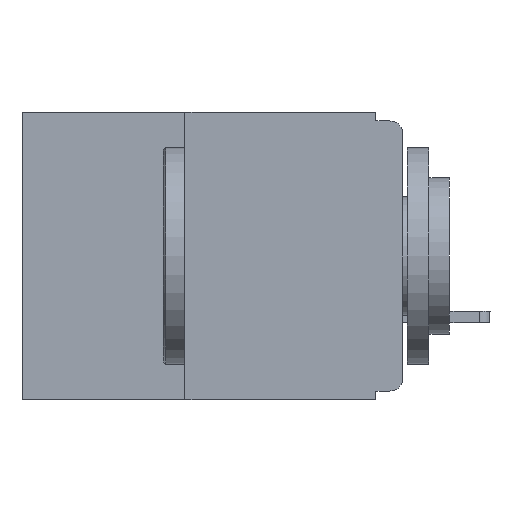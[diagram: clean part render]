
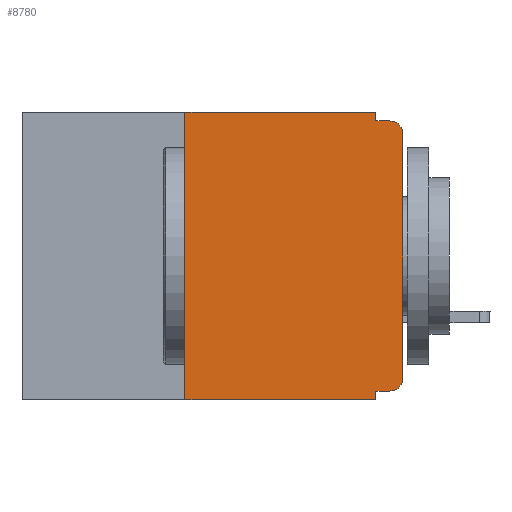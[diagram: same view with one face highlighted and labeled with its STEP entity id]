
A CAD part, left-side view. The second image highlights one B-rep face of the part: STEP entity #8780.
In plain terms, the highlighted planar face has unit normal (-1, 0, 0).
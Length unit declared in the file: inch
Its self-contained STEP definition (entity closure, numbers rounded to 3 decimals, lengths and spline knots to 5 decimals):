
#57 = VECTOR ( 'NONE', #1416, 39.37008 ) ;
#138 = DIRECTION ( 'NONE',  ( 0., 0., -1. ) ) ;
#514 = DIRECTION ( 'NONE',  ( 0., -1., 0. ) ) ;
#911 = CARTESIAN_POINT ( 'NONE',  ( 0., 0.031, 0. ) ) ;
#1019 = PLANE ( 'NONE',  #12183 ) ;
#1063 = CARTESIAN_POINT ( 'NONE',  ( 0., 0., -0.305 ) ) ;
#1416 = DIRECTION ( 'NONE',  ( 0., -1., 0. ) ) ;
#1552 = CARTESIAN_POINT ( 'NONE',  ( 0., 0.031, -0.33 ) ) ;
#1625 = AXIS2_PLACEMENT_3D ( 'NONE', #15796, #3561, #138 ) ;
#1792 = LINE ( 'NONE', #9131, #11080 ) ;
#1931 = VECTOR ( 'NONE', #14761, 39.37008 ) ;
#1936 = EDGE_CURVE ( 'NONE', #6813, #5561, #2274, .T. ) ;
#2003 = LINE ( 'NONE', #6343, #3177 ) ;
#2274 = LINE ( 'NONE', #7896, #9621 ) ;
#2486 = DIRECTION ( 'NONE',  ( 0., 0., -1. ) ) ;
#2581 = CARTESIAN_POINT ( 'NONE',  ( 0., 0.25, -0.33 ) ) ;
#2780 = VERTEX_POINT ( 'NONE', #13737 ) ;
#2815 = ORIENTED_EDGE ( 'NONE', *, *, #11967, .F. ) ;
#2892 = EDGE_CURVE ( 'NONE', #4683, #4718, #8689, .T. ) ;
#3177 = VECTOR ( 'NONE', #15014, 39.37008 ) ;
#3210 = EDGE_CURVE ( 'NONE', #4718, #3398, #5252, .T. ) ;
#3268 = EDGE_CURVE ( 'NONE', #3398, #5561, #15528, .T. ) ;
#3398 = VERTEX_POINT ( 'NONE', #6577 ) ;
#3561 = DIRECTION ( 'NONE',  ( -1., 0., 0. ) ) ;
#4057 = ORIENTED_EDGE ( 'NONE', *, *, #3210, .T. ) ;
#4130 = EDGE_CURVE ( 'NONE', #9126, #6813, #12400, .T. ) ;
#4626 = AXIS2_PLACEMENT_3D ( 'NONE', #12476, #7339, #8658 ) ;
#4683 = VERTEX_POINT ( 'NONE', #12963 ) ;
#4718 = VERTEX_POINT ( 'NONE', #1063 ) ;
#5240 = LINE ( 'NONE', #2581, #1931 ) ;
#5252 = LINE ( 'NONE', #10010, #13376 ) ;
#5350 = CARTESIAN_POINT ( 'NONE',  ( 0., 0.031, 0. ) ) ;
#5561 = VERTEX_POINT ( 'NONE', #12480 ) ;
#5664 = VERTEX_POINT ( 'NONE', #1552 ) ;
#6192 = VERTEX_POINT ( 'NONE', #11541 ) ;
#6343 = CARTESIAN_POINT ( 'NONE',  ( 0., 0.031, -0.33 ) ) ;
#6577 = CARTESIAN_POINT ( 'NONE',  ( 0., 0., -0.025 ) ) ;
#6813 = VERTEX_POINT ( 'NONE', #14685 ) ;
#7339 = DIRECTION ( 'NONE',  ( -1., 0., 0. ) ) ;
#7783 = EDGE_LOOP ( 'NONE', ( #4057, #12199, #14341, #14752, #15114, #13773, #15693, #15329, #2815, #10581 ) ) ;
#7896 = CARTESIAN_POINT ( 'NONE',  ( 0., 0., -0.01 ) ) ;
#7956 = CARTESIAN_POINT ( 'NONE',  ( 0., 0., -0.32 ) ) ;
#8032 = VERTEX_POINT ( 'NONE', #9036 ) ;
#8658 = DIRECTION ( 'NONE',  ( 0., 0., -1. ) ) ;
#8689 = CIRCLE ( 'NONE', #1625, 0.015 ) ;
#8780 = ADVANCED_FACE ( 'NONE', ( #12027 ), #1019, .F. ) ;
#8816 = DIRECTION ( 'NONE',  ( 0., 0., 1. ) ) ;
#9036 = CARTESIAN_POINT ( 'NONE',  ( 0., 0.25, 0. ) ) ;
#9043 = EDGE_CURVE ( 'NONE', #6192, #5664, #1792, .T. ) ;
#9126 = VERTEX_POINT ( 'NONE', #5350 ) ;
#9131 = CARTESIAN_POINT ( 'NONE',  ( 0., 0.437, -0.33 ) ) ;
#9141 = DIRECTION ( 'NONE',  ( 0., 1., 0. ) ) ;
#9314 = LINE ( 'NONE', #7956, #10870 ) ;
#9581 = DIRECTION ( 'NONE',  ( 0., 0., -1. ) ) ;
#9621 = VECTOR ( 'NONE', #514, 39.37008 ) ;
#9746 = DIRECTION ( 'NONE',  ( 1., 0., 0. ) ) ;
#10010 = CARTESIAN_POINT ( 'NONE',  ( 0., 0., 0. ) ) ;
#10207 = DIRECTION ( 'NONE',  ( 0., -1., 0. ) ) ;
#10555 = EDGE_CURVE ( 'NONE', #2780, #5664, #2003, .T. ) ;
#10581 = ORIENTED_EDGE ( 'NONE', *, *, #2892, .T. ) ;
#10870 = VECTOR ( 'NONE', #9141, 39.37008 ) ;
#11080 = VECTOR ( 'NONE', #10207, 39.37008 ) ;
#11097 = LINE ( 'NONE', #14678, #57 ) ;
#11312 = EDGE_CURVE ( 'NONE', #8032, #9126, #11097, .T. ) ;
#11541 = CARTESIAN_POINT ( 'NONE',  ( 0., 0.25, -0.33 ) ) ;
#11967 = EDGE_CURVE ( 'NONE', #4683, #2780, #9314, .T. ) ;
#12027 = FACE_OUTER_BOUND ( 'NONE', #7783, .T. ) ;
#12183 = AXIS2_PLACEMENT_3D ( 'NONE', #14775, #9746, #2486 ) ;
#12197 = VECTOR ( 'NONE', #9581, 39.37008 ) ;
#12199 = ORIENTED_EDGE ( 'NONE', *, *, #3268, .T. ) ;
#12279 = EDGE_CURVE ( 'NONE', #6192, #8032, #5240, .T. ) ;
#12400 = LINE ( 'NONE', #911, #12197 ) ;
#12476 = CARTESIAN_POINT ( 'NONE',  ( 0., 0.015, -0.025 ) ) ;
#12480 = CARTESIAN_POINT ( 'NONE',  ( 0., 0.015, -0.01 ) ) ;
#12963 = CARTESIAN_POINT ( 'NONE',  ( 0., 0.015, -0.32 ) ) ;
#13376 = VECTOR ( 'NONE', #8816, 39.37008 ) ;
#13737 = CARTESIAN_POINT ( 'NONE',  ( 0., 0.031, -0.32 ) ) ;
#13773 = ORIENTED_EDGE ( 'NONE', *, *, #12279, .F. ) ;
#14341 = ORIENTED_EDGE ( 'NONE', *, *, #1936, .F. ) ;
#14678 = CARTESIAN_POINT ( 'NONE',  ( 0., 0.437, 0. ) ) ;
#14685 = CARTESIAN_POINT ( 'NONE',  ( 0., 0.031, -0.01 ) ) ;
#14752 = ORIENTED_EDGE ( 'NONE', *, *, #4130, .F. ) ;
#14761 = DIRECTION ( 'NONE',  ( 0., 0., 1. ) ) ;
#14775 = CARTESIAN_POINT ( 'NONE',  ( 0., 0.437, 0. ) ) ;
#15014 = DIRECTION ( 'NONE',  ( 0., 0., -1. ) ) ;
#15114 = ORIENTED_EDGE ( 'NONE', *, *, #11312, .F. ) ;
#15329 = ORIENTED_EDGE ( 'NONE', *, *, #10555, .F. ) ;
#15528 = CIRCLE ( 'NONE', #4626, 0.015 ) ;
#15693 = ORIENTED_EDGE ( 'NONE', *, *, #9043, .T. ) ;
#15796 = CARTESIAN_POINT ( 'NONE',  ( 0., 0.015, -0.305 ) ) ;
